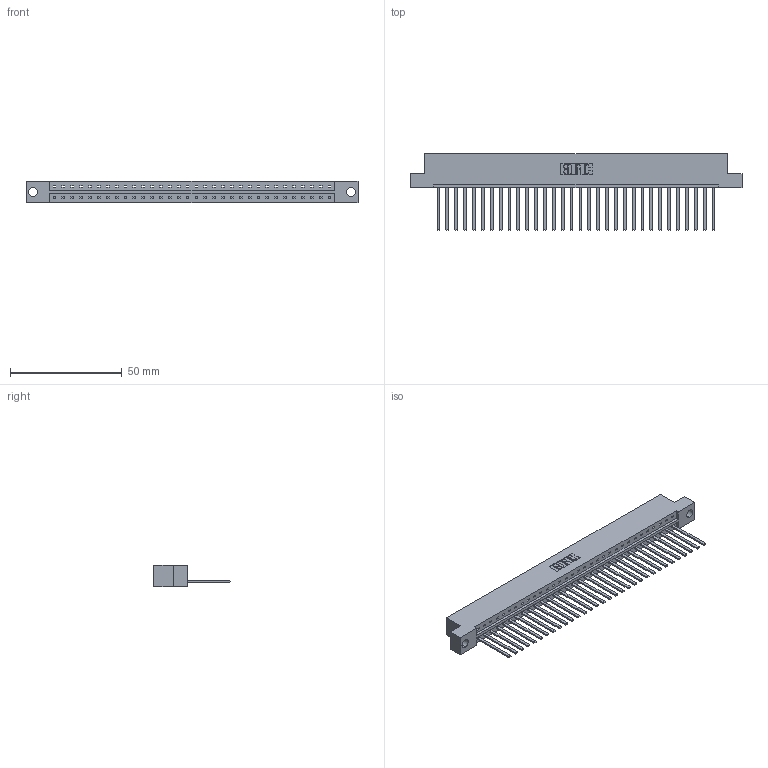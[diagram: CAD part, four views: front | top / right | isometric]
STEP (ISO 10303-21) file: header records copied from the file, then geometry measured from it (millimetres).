
FILE_DESCRIPTION (( 'STEP AP203' ), '1' );
FILE_NAME ('833-032-544-104.STEP', '2020-06-02T18:38:25', ( '' ), ( '' ), 'SwSTEP 2.0', 'SolidWorks 2020', '' );
FILE_SCHEMA (( 'CONFIG_CONTROL_DESIGN' ));
Length unit declared in the file: inch
Products named in the file (3): 345-292-001_345-293-144; 833-032-544-104; 833 Part_Flush - .156 Dia - TH
Assembly tree (33 placements, depth 2):
  833-032-544-104
    833 Part_Flush - .156 Dia - TH
    345-292-001_345-293-144  x32
Bounding box: 148.34 x 34.3 x 9.4 mm (x, y, z)
Volume: 15123.5 mm3; surface area: 17298.4 mm2
Topology: 33 solids, 33 shells, 1778 faces, 5367 edges, 3534 vertices
Faces by surface type: plane 1286, cylinder 492
Entity records: 20675 total; most frequent: CARTESIAN_POINT 3574, ORIENTED_EDGE 3542, DIRECTION 3031, EDGE_CURVE 1771, VECTOR 1647, LINE 1647, VERTEX_POINT 1178, AXIS2_PLACEMENT_3D 692
